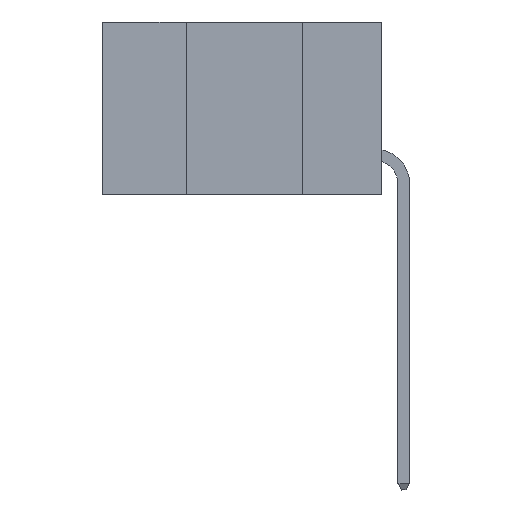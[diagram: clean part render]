
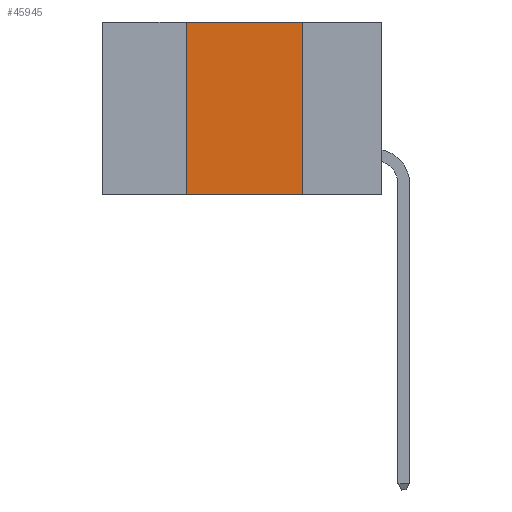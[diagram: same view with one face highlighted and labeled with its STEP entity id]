
A CAD part, left-side view. The second image highlights one B-rep face of the part: STEP entity #45945.
In plain terms, the highlighted planar face has unit normal (-1, 0, 0).
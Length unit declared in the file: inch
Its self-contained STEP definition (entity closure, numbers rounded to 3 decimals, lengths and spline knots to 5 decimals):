
#22 = CARTESIAN_POINT ( 'NONE',  ( 0., 0.42, 0. ) ) ;
#2172 = VERTEX_POINT ( 'NONE', #4195 ) ;
#4195 = CARTESIAN_POINT ( 'NONE',  ( 0., 0.17, 0. ) ) ;
#6372 = VERTEX_POINT ( 'NONE', #22 ) ;
#6961 = CARTESIAN_POINT ( 'NONE',  ( 0., 0.6, 0. ) ) ;
#7125 = PLANE ( 'NONE',  #19638 ) ;
#7950 = VECTOR ( 'NONE', #31028, 39.37008 ) ;
#8222 = LINE ( 'NONE', #38445, #35811 ) ;
#10055 = DIRECTION ( 'NONE',  ( 0., 0., 1. ) ) ;
#11180 = CARTESIAN_POINT ( 'NONE',  ( 0., 0.17, -0.37 ) ) ;
#11621 = VECTOR ( 'NONE', #10055, 39.37008 ) ;
#11728 = EDGE_CURVE ( 'NONE', #45540, #28850, #8222, .T. ) ;
#13046 = DIRECTION ( 'NONE',  ( 0., 0., -1. ) ) ;
#13630 = CARTESIAN_POINT ( 'NONE',  ( 0., 0.42, 0. ) ) ;
#17186 = VECTOR ( 'NONE', #13046, 39.37008 ) ;
#18436 = ORIENTED_EDGE ( 'NONE', *, *, #19642, .F. ) ;
#19638 = AXIS2_PLACEMENT_3D ( 'NONE', #6961, #44583, #29140 ) ;
#19642 = EDGE_CURVE ( 'NONE', #2172, #28850, #37168, .T. ) ;
#19880 = CARTESIAN_POINT ( 'NONE',  ( 0., 0.6, 0. ) ) ;
#26869 = LINE ( 'NONE', #13630, #11621 ) ;
#27894 = LINE ( 'NONE', #19880, #7950 ) ;
#28850 = VERTEX_POINT ( 'NONE', #11180 ) ;
#29140 = DIRECTION ( 'NONE',  ( 0., 0., -1. ) ) ;
#30739 = EDGE_LOOP ( 'NONE', ( #18436, #32865, #35575, #41748 ) ) ;
#31028 = DIRECTION ( 'NONE',  ( 0., -1., 0. ) ) ;
#31465 = CARTESIAN_POINT ( 'NONE',  ( 0., 0.42, -0.37 ) ) ;
#32090 = CARTESIAN_POINT ( 'NONE',  ( 0., 0.17, 0. ) ) ;
#32865 = ORIENTED_EDGE ( 'NONE', *, *, #46122, .F. ) ;
#34328 = DIRECTION ( 'NONE',  ( 0., -1., 0. ) ) ;
#34365 = FACE_OUTER_BOUND ( 'NONE', #30739, .T. ) ;
#35575 = ORIENTED_EDGE ( 'NONE', *, *, #47302, .F. ) ;
#35811 = VECTOR ( 'NONE', #34328, 39.37008 ) ;
#37168 = LINE ( 'NONE', #32090, #17186 ) ;
#38445 = CARTESIAN_POINT ( 'NONE',  ( 0., 0.6, -0.37 ) ) ;
#41748 = ORIENTED_EDGE ( 'NONE', *, *, #11728, .T. ) ;
#44583 = DIRECTION ( 'NONE',  ( 1., 0., 0. ) ) ;
#45540 = VERTEX_POINT ( 'NONE', #31465 ) ;
#45945 = ADVANCED_FACE ( 'NONE', ( #34365 ), #7125, .F. ) ;
#46122 = EDGE_CURVE ( 'NONE', #6372, #2172, #27894, .T. ) ;
#47302 = EDGE_CURVE ( 'NONE', #45540, #6372, #26869, .T. ) ;
